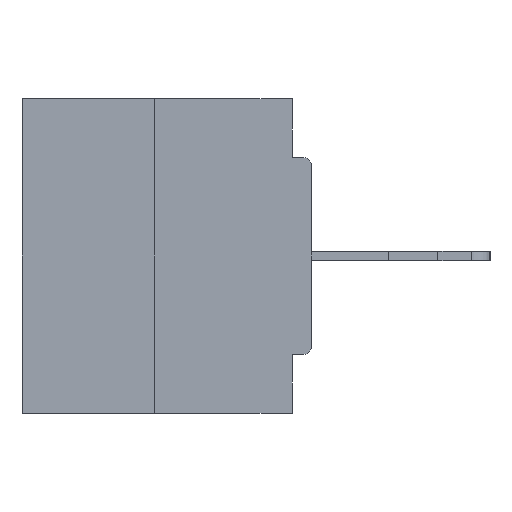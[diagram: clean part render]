
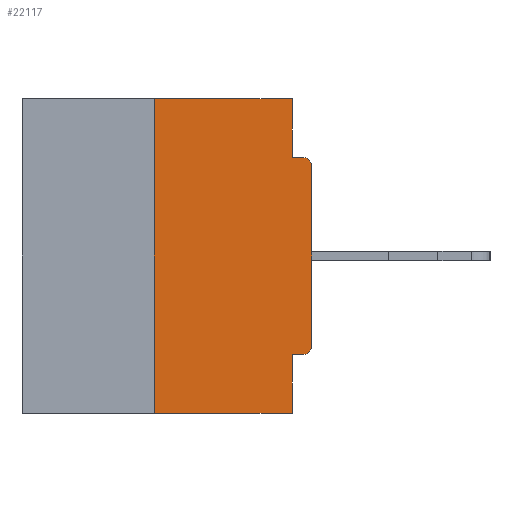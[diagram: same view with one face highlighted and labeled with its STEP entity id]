
A CAD part, left-side view. The second image highlights one B-rep face of the part: STEP entity #22117.
In plain terms, the highlighted planar face has unit normal (-1, 0, 0).
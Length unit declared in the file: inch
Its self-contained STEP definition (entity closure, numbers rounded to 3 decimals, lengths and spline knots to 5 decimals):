
#9 = DIRECTION ( 'NONE',  ( 0., 0., -1. ) ) ;
#205 = CARTESIAN_POINT ( 'NONE',  ( 0., 0.25, 0. ) ) ;
#236 = VERTEX_POINT ( 'NONE', #16974 ) ;
#346 = CARTESIAN_POINT ( 'NONE',  ( 0., 0.46, -0.5 ) ) ;
#354 = CARTESIAN_POINT ( 'NONE',  ( 0., 0.46, 0. ) ) ;
#515 = AXIS2_PLACEMENT_3D ( 'NONE', #20988, #12459, #7988 ) ;
#1061 = VERTEX_POINT ( 'NONE', #8742 ) ;
#1208 = DIRECTION ( 'NONE',  ( 0., 0., 1. ) ) ;
#1768 = VECTOR ( 'NONE', #16201, 39.37008 ) ;
#1809 = VECTOR ( 'NONE', #8732, 39.37008 ) ;
#2148 = AXIS2_PLACEMENT_3D ( 'NONE', #22975, #11742, #20725 ) ;
#2231 = ORIENTED_EDGE ( 'NONE', *, *, #18187, .F. ) ;
#2471 = DIRECTION ( 'NONE',  ( 0., -1., 0. ) ) ;
#3417 = CARTESIAN_POINT ( 'NONE',  ( 0., 0., -0.0935 ) ) ;
#3501 = VERTEX_POINT ( 'NONE', #26878 ) ;
#3607 = EDGE_CURVE ( 'NONE', #236, #3501, #7593, .T. ) ;
#3893 = EDGE_CURVE ( 'NONE', #23529, #23735, #15749, .T. ) ;
#4297 = EDGE_CURVE ( 'NONE', #26806, #20065, #22870, .T. ) ;
#5481 = EDGE_CURVE ( 'NONE', #27080, #12652, #9151, .T. ) ;
#5630 = FACE_OUTER_BOUND ( 'NONE', #27584, .T. ) ;
#6969 = CIRCLE ( 'NONE', #16407, 0.015 ) ;
#7593 = LINE ( 'NONE', #12500, #17761 ) ;
#7988 = DIRECTION ( 'NONE',  ( 0., 0., -1. ) ) ;
#8237 = CARTESIAN_POINT ( 'NONE',  ( 0., 0.25, -0.5 ) ) ;
#8732 = DIRECTION ( 'NONE',  ( 0., 0., -1. ) ) ;
#8742 = CARTESIAN_POINT ( 'NONE',  ( 0., 0.031, -0.0935 ) ) ;
#9151 = LINE ( 'NONE', #354, #15365 ) ;
#9479 = DIRECTION ( 'NONE',  ( 0., 0., 1. ) ) ;
#10108 = PLANE ( 'NONE',  #515 ) ;
#10202 = CARTESIAN_POINT ( 'NONE',  ( 0., 0.031, 0. ) ) ;
#10533 = EDGE_CURVE ( 'NONE', #12652, #1061, #11303, .T. ) ;
#11027 = ORIENTED_EDGE ( 'NONE', *, *, #10533, .F. ) ;
#11303 = LINE ( 'NONE', #20281, #17005 ) ;
#11535 = CARTESIAN_POINT ( 'NONE',  ( 0., 0.031, -0.5 ) ) ;
#11742 = DIRECTION ( 'NONE',  ( -1., 0., 0. ) ) ;
#12222 = CARTESIAN_POINT ( 'NONE',  ( 0., 0.031, -0.4065 ) ) ;
#12459 = DIRECTION ( 'NONE',  ( 1., 0., 0. ) ) ;
#12473 = DIRECTION ( 'NONE',  ( 0., -1., 0. ) ) ;
#12500 = CARTESIAN_POINT ( 'NONE',  ( 0., 0., 0. ) ) ;
#12652 = VERTEX_POINT ( 'NONE', #10202 ) ;
#12992 = ORIENTED_EDGE ( 'NONE', *, *, #3893, .F. ) ;
#13020 = CIRCLE ( 'NONE', #2148, 0.015 ) ;
#13323 = LINE ( 'NONE', #11535, #1809 ) ;
#13690 = DIRECTION ( 'NONE',  ( 0., 1., 0. ) ) ;
#14491 = LINE ( 'NONE', #23492, #26886 ) ;
#14629 = ORIENTED_EDGE ( 'NONE', *, *, #17391, .T. ) ;
#14659 = LINE ( 'NONE', #3417, #28249 ) ;
#15280 = EDGE_CURVE ( 'NONE', #3501, #16947, #13020, .T. ) ;
#15365 = VECTOR ( 'NONE', #2471, 39.37008 ) ;
#15465 = ORIENTED_EDGE ( 'NONE', *, *, #4297, .T. ) ;
#15749 = LINE ( 'NONE', #15885, #28728 ) ;
#15885 = CARTESIAN_POINT ( 'NONE',  ( 0., 0., -0.4065 ) ) ;
#16020 = CARTESIAN_POINT ( 'NONE',  ( 0., 0.015, -0.0935 ) ) ;
#16126 = ORIENTED_EDGE ( 'NONE', *, *, #5481, .F. ) ;
#16201 = DIRECTION ( 'NONE',  ( 0., -1., 0. ) ) ;
#16407 = AXIS2_PLACEMENT_3D ( 'NONE', #20651, #27498, #18457 ) ;
#16947 = VERTEX_POINT ( 'NONE', #16020 ) ;
#16974 = CARTESIAN_POINT ( 'NONE',  ( 0., 0., -0.3915 ) ) ;
#17005 = VECTOR ( 'NONE', #9, 39.37008 ) ;
#17391 = EDGE_CURVE ( 'NONE', #23529, #236, #6969, .T. ) ;
#17761 = VECTOR ( 'NONE', #1208, 39.37008 ) ;
#18187 = EDGE_CURVE ( 'NONE', #26806, #27080, #14491, .T. ) ;
#18457 = DIRECTION ( 'NONE',  ( 0., 0., -1. ) ) ;
#18916 = EDGE_CURVE ( 'NONE', #1061, #16947, #14659, .T. ) ;
#19597 = EDGE_CURVE ( 'NONE', #23735, #20065, #13323, .T. ) ;
#19883 = CARTESIAN_POINT ( 'NONE',  ( 0., 0.031, -0.5 ) ) ;
#20065 = VERTEX_POINT ( 'NONE', #19883 ) ;
#20281 = CARTESIAN_POINT ( 'NONE',  ( 0., 0.031, 0. ) ) ;
#20651 = CARTESIAN_POINT ( 'NONE',  ( 0., 0.015, -0.3915 ) ) ;
#20725 = DIRECTION ( 'NONE',  ( 0., 0., -1. ) ) ;
#20988 = CARTESIAN_POINT ( 'NONE',  ( 0., 0.46, 0. ) ) ;
#22117 = ADVANCED_FACE ( 'NONE', ( #5630 ), #10108, .F. ) ;
#22870 = LINE ( 'NONE', #346, #1768 ) ;
#22967 = ORIENTED_EDGE ( 'NONE', *, *, #18916, .F. ) ;
#22975 = CARTESIAN_POINT ( 'NONE',  ( 0., 0.015, -0.1085 ) ) ;
#23492 = CARTESIAN_POINT ( 'NONE',  ( 0., 0.25, 0. ) ) ;
#23529 = VERTEX_POINT ( 'NONE', #23853 ) ;
#23735 = VERTEX_POINT ( 'NONE', #12222 ) ;
#23853 = CARTESIAN_POINT ( 'NONE',  ( 0., 0.015, -0.4065 ) ) ;
#26806 = VERTEX_POINT ( 'NONE', #8237 ) ;
#26878 = CARTESIAN_POINT ( 'NONE',  ( 0., 0., -0.1085 ) ) ;
#26886 = VECTOR ( 'NONE', #9479, 39.37008 ) ;
#27080 = VERTEX_POINT ( 'NONE', #205 ) ;
#27498 = DIRECTION ( 'NONE',  ( -1., 0., 0. ) ) ;
#27584 = EDGE_LOOP ( 'NONE', ( #16126, #2231, #15465, #28664, #12992, #14629, #27908, #28672, #22967, #11027 ) ) ;
#27908 = ORIENTED_EDGE ( 'NONE', *, *, #3607, .T. ) ;
#28249 = VECTOR ( 'NONE', #12473, 39.37008 ) ;
#28664 = ORIENTED_EDGE ( 'NONE', *, *, #19597, .F. ) ;
#28672 = ORIENTED_EDGE ( 'NONE', *, *, #15280, .T. ) ;
#28728 = VECTOR ( 'NONE', #13690, 39.37008 ) ;
